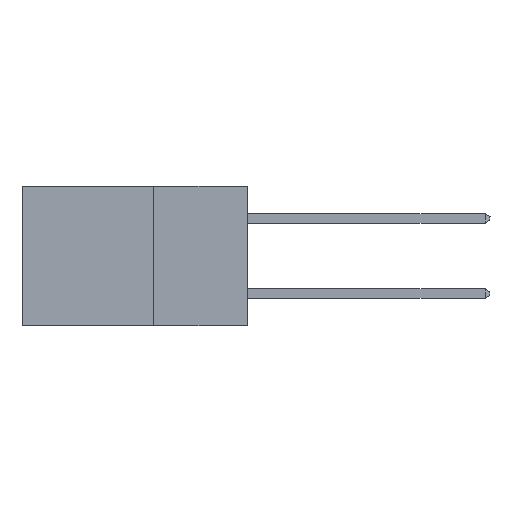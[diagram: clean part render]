
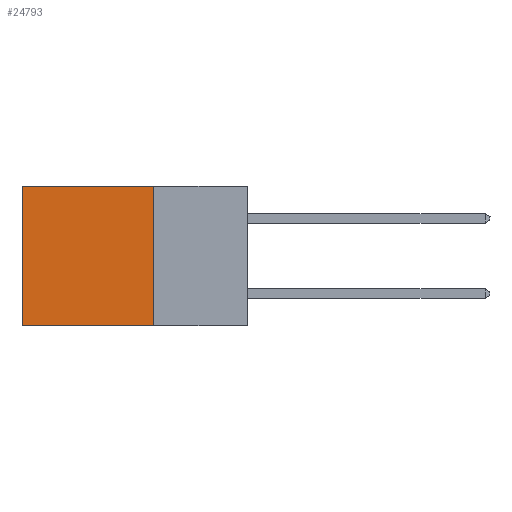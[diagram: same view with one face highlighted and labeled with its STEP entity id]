
A CAD part, left-side view. The second image highlights one B-rep face of the part: STEP entity #24793.
In plain terms, the highlighted planar face has unit normal (-1, 0, 0).
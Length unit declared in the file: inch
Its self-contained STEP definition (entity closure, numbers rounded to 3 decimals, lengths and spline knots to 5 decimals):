
#1240 = DIRECTION ( 'NONE',  ( 0., 1., 0. ) ) ;
#1410 = CARTESIAN_POINT ( 'NONE',  ( 0.298, 0.25, 0. ) ) ;
#1642 = EDGE_CURVE ( 'NONE', #6880, #22355, #5075, .T. ) ;
#3940 = DIRECTION ( 'NONE',  ( 0., 1., 0. ) ) ;
#5075 = LINE ( 'NONE', #25909, #27048 ) ;
#6880 = VERTEX_POINT ( 'NONE', #11791 ) ;
#9812 = EDGE_LOOP ( 'NONE', ( #23758, #10747, #9845, #19185 ) ) ;
#9845 = ORIENTED_EDGE ( 'NONE', *, *, #12803, .F. ) ;
#10747 = ORIENTED_EDGE ( 'NONE', *, *, #1642, .F. ) ;
#11791 = CARTESIAN_POINT ( 'NONE',  ( 0.298, 0.25, -0.37 ) ) ;
#11982 = CARTESIAN_POINT ( 'NONE',  ( 0.298, 0.6, -0.37 ) ) ;
#12151 = DIRECTION ( 'NONE',  ( 1., 0., 0. ) ) ;
#12803 = EDGE_CURVE ( 'NONE', #16556, #6880, #28981, .T. ) ;
#12997 = CARTESIAN_POINT ( 'NONE',  ( 0.298, 0.6, 0. ) ) ;
#13352 = LINE ( 'NONE', #17649, #16541 ) ;
#13552 = CARTESIAN_POINT ( 'NONE',  ( 0.298, 0.25, 0. ) ) ;
#14680 = VERTEX_POINT ( 'NONE', #12997 ) ;
#16541 = VECTOR ( 'NONE', #24484, 39.37008 ) ;
#16549 = VECTOR ( 'NONE', #29245, 39.37008 ) ;
#16556 = VERTEX_POINT ( 'NONE', #1410 ) ;
#16868 = FACE_OUTER_BOUND ( 'NONE', #9812, .T. ) ;
#17459 = CARTESIAN_POINT ( 'NONE',  ( 0.298, 0.25, 0. ) ) ;
#17649 = CARTESIAN_POINT ( 'NONE',  ( 0.298, 0.6, 0. ) ) ;
#19066 = VECTOR ( 'NONE', #3940, 39.37008 ) ;
#19179 = PLANE ( 'NONE',  #22652 ) ;
#19185 = ORIENTED_EDGE ( 'NONE', *, *, #23570, .T. ) ;
#20233 = EDGE_CURVE ( 'NONE', #14680, #22355, #13352, .T. ) ;
#21143 = CARTESIAN_POINT ( 'NONE',  ( 0.298, 0.25, 0. ) ) ;
#22355 = VERTEX_POINT ( 'NONE', #11982 ) ;
#22652 = AXIS2_PLACEMENT_3D ( 'NONE', #21143, #12151, #23466 ) ;
#23466 = DIRECTION ( 'NONE',  ( 0., 0., -1. ) ) ;
#23570 = EDGE_CURVE ( 'NONE', #16556, #14680, #25077, .T. ) ;
#23758 = ORIENTED_EDGE ( 'NONE', *, *, #20233, .T. ) ;
#24484 = DIRECTION ( 'NONE',  ( 0., 0., -1. ) ) ;
#24793 = ADVANCED_FACE ( 'NONE', ( #16868 ), #19179, .F. ) ;
#25077 = LINE ( 'NONE', #17459, #19066 ) ;
#25909 = CARTESIAN_POINT ( 'NONE',  ( 0.298, 0.25, -0.37 ) ) ;
#27048 = VECTOR ( 'NONE', #1240, 39.37008 ) ;
#28981 = LINE ( 'NONE', #13552, #16549 ) ;
#29245 = DIRECTION ( 'NONE',  ( 0., 0., -1. ) ) ;
